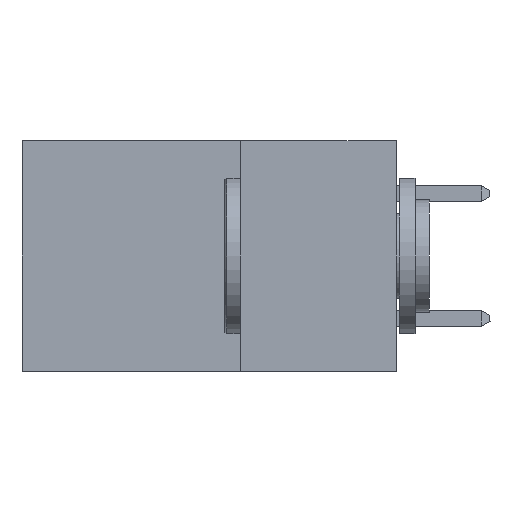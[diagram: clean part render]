
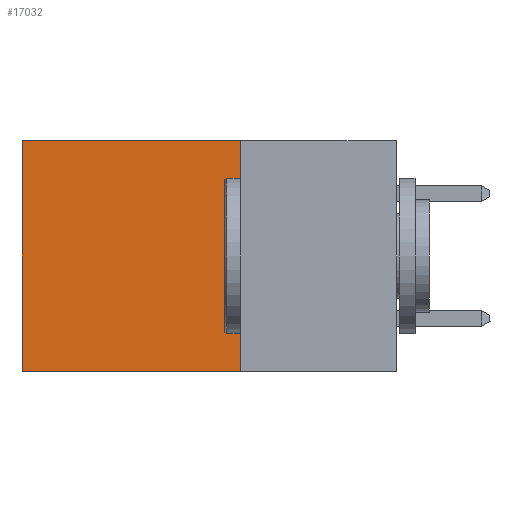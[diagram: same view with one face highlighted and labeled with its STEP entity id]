
A CAD part, left-side view. The second image highlights one B-rep face of the part: STEP entity #17032.
In plain terms, the highlighted planar face has unit normal (-1, 0, 0).
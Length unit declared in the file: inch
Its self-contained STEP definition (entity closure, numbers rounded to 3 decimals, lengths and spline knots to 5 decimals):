
#1573 = VECTOR ( 'NONE', #19036, 39.37008 ) ;
#1786 = DIRECTION ( 'NONE',  ( 0., 0., -1. ) ) ;
#2595 = CARTESIAN_POINT ( 'NONE',  ( 0.298, 0.25, 0. ) ) ;
#3033 = ORIENTED_EDGE ( 'NONE', *, *, #8259, .F. ) ;
#3177 = VERTEX_POINT ( 'NONE', #8325 ) ;
#3703 = DIRECTION ( 'NONE',  ( 1., 0., 0. ) ) ;
#3990 = VERTEX_POINT ( 'NONE', #2595 ) ;
#5067 = LINE ( 'NONE', #7681, #19568 ) ;
#6407 = DIRECTION ( 'NONE',  ( 0., 1., 0. ) ) ;
#7204 = EDGE_LOOP ( 'NONE', ( #12241, #21656, #3033, #19730 ) ) ;
#7681 = CARTESIAN_POINT ( 'NONE',  ( 0.298, 0.6, 0. ) ) ;
#8259 = EDGE_CURVE ( 'NONE', #3990, #17804, #16627, .T. ) ;
#8325 = CARTESIAN_POINT ( 'NONE',  ( 0.298, 0.6, 0. ) ) ;
#8344 = CARTESIAN_POINT ( 'NONE',  ( 0.298, 0.25, -0.37 ) ) ;
#8449 = FACE_OUTER_BOUND ( 'NONE', #7204, .T. ) ;
#8658 = CARTESIAN_POINT ( 'NONE',  ( 0.298, 0.6, -0.37 ) ) ;
#9317 = VERTEX_POINT ( 'NONE', #8658 ) ;
#11033 = EDGE_CURVE ( 'NONE', #3177, #9317, #5067, .T. ) ;
#11665 = CARTESIAN_POINT ( 'NONE',  ( 0.298, 0.25, 0. ) ) ;
#11836 = LINE ( 'NONE', #17087, #1573 ) ;
#12241 = ORIENTED_EDGE ( 'NONE', *, *, #11033, .T. ) ;
#12671 = VECTOR ( 'NONE', #25243, 39.37008 ) ;
#15962 = EDGE_CURVE ( 'NONE', #17804, #9317, #23783, .T. ) ;
#16627 = LINE ( 'NONE', #11665, #12671 ) ;
#17032 = ADVANCED_FACE ( 'NONE', ( #8449 ), #21383, .F. ) ;
#17087 = CARTESIAN_POINT ( 'NONE',  ( 0.298, 0.25, 0. ) ) ;
#17554 = DIRECTION ( 'NONE',  ( 0., 0., -1. ) ) ;
#17804 = VERTEX_POINT ( 'NONE', #8344 ) ;
#18194 = CARTESIAN_POINT ( 'NONE',  ( 0.298, 0.25, -0.37 ) ) ;
#19036 = DIRECTION ( 'NONE',  ( 0., 1., 0. ) ) ;
#19568 = VECTOR ( 'NONE', #1786, 39.37008 ) ;
#19730 = ORIENTED_EDGE ( 'NONE', *, *, #25251, .T. ) ;
#21383 = PLANE ( 'NONE',  #22414 ) ;
#21656 = ORIENTED_EDGE ( 'NONE', *, *, #15962, .F. ) ;
#22414 = AXIS2_PLACEMENT_3D ( 'NONE', #25267, #3703, #17554 ) ;
#23186 = VECTOR ( 'NONE', #6407, 39.37008 ) ;
#23783 = LINE ( 'NONE', #18194, #23186 ) ;
#25243 = DIRECTION ( 'NONE',  ( 0., 0., -1. ) ) ;
#25251 = EDGE_CURVE ( 'NONE', #3990, #3177, #11836, .T. ) ;
#25267 = CARTESIAN_POINT ( 'NONE',  ( 0.298, 0.25, 0. ) ) ;
